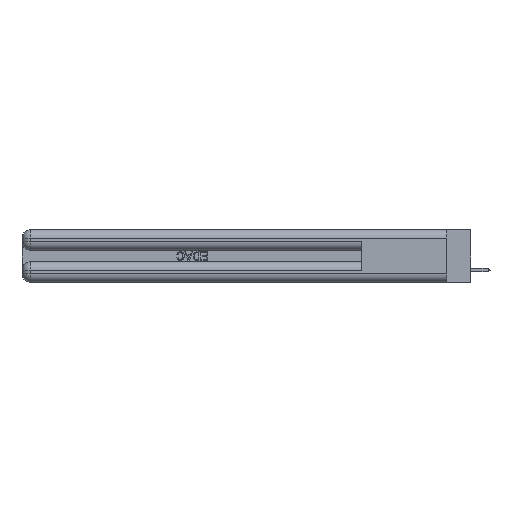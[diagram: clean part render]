
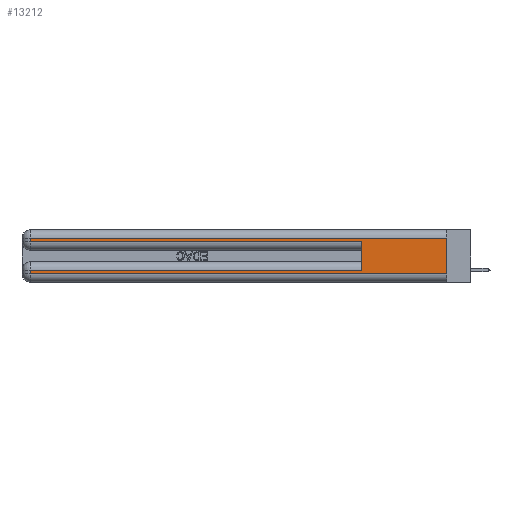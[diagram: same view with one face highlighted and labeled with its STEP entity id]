
A CAD part, left-side view. The second image highlights one B-rep face of the part: STEP entity #13212.
In plain terms, the highlighted planar face has unit normal (-1, 0, 0).
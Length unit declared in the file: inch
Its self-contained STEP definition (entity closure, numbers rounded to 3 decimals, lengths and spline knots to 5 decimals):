
#26 = EDGE_LOOP ( 'NONE', ( #48229, #40978, #5168, #26875, #28088, #43098, #944, #20718 ) ) ;
#944 = ORIENTED_EDGE ( 'NONE', *, *, #6880, .T. ) ;
#1150 = DIRECTION ( 'NONE',  ( 0., 0., -1. ) ) ;
#1987 = VECTOR ( 'NONE', #1150, 39.37008 ) ;
#2063 = EDGE_CURVE ( 'NONE', #20441, #38896, #4569, .T. ) ;
#2819 = EDGE_CURVE ( 'NONE', #20441, #10997, #40983, .T. ) ;
#4569 = LINE ( 'NONE', #18799, #24946 ) ;
#5143 = DIRECTION ( 'NONE',  ( 0., 1., 0. ) ) ;
#5168 = ORIENTED_EDGE ( 'NONE', *, *, #30772, .T. ) ;
#6452 = LINE ( 'NONE', #38888, #9509 ) ;
#6711 = EDGE_CURVE ( 'NONE', #26105, #38896, #39198, .T. ) ;
#6880 = EDGE_CURVE ( 'NONE', #10997, #44248, #21819, .T. ) ;
#7583 = VERTEX_POINT ( 'NONE', #15220 ) ;
#7805 = PLANE ( 'NONE',  #35857 ) ;
#7913 = DIRECTION ( 'NONE',  ( 0., 0., 1. ) ) ;
#7926 = CARTESIAN_POINT ( 'NONE',  ( 0., 2.94, 0.085 ) ) ;
#8089 = DIRECTION ( 'NONE',  ( 0., -1., 0. ) ) ;
#8576 = DIRECTION ( 'NONE',  ( 0., -1., 0. ) ) ;
#9509 = VECTOR ( 'NONE', #20140, 39.37008 ) ;
#10997 = VERTEX_POINT ( 'NONE', #7926 ) ;
#11339 = CARTESIAN_POINT ( 'NONE',  ( 0., 0., 0.31 ) ) ;
#13212 = ADVANCED_FACE ( 'NONE', ( #26856 ), #7805, .F. ) ;
#14032 = CARTESIAN_POINT ( 'NONE',  ( 0., 2.94, 0.285 ) ) ;
#15220 = CARTESIAN_POINT ( 'NONE',  ( 0., 2.94, 0.31 ) ) ;
#18799 = CARTESIAN_POINT ( 'NONE',  ( 0., 0.6, 0.145 ) ) ;
#18947 = VECTOR ( 'NONE', #5143, 39.37008 ) ;
#19953 = LINE ( 'NONE', #28258, #47176 ) ;
#19994 = DIRECTION ( 'NONE',  ( 0., 1., 0. ) ) ;
#20140 = DIRECTION ( 'NONE',  ( 0., 0., -1. ) ) ;
#20441 = VERTEX_POINT ( 'NONE', #39815 ) ;
#20532 = VECTOR ( 'NONE', #19994, 39.37008 ) ;
#20718 = ORIENTED_EDGE ( 'NONE', *, *, #27143, .T. ) ;
#21819 = LINE ( 'NONE', #34352, #29849 ) ;
#22660 = CARTESIAN_POINT ( 'NONE',  ( 0., 2.94, 0.06 ) ) ;
#24946 = VECTOR ( 'NONE', #7913, 39.37008 ) ;
#26105 = VERTEX_POINT ( 'NONE', #14032 ) ;
#26856 = FACE_OUTER_BOUND ( 'NONE', #26, .T. ) ;
#26875 = ORIENTED_EDGE ( 'NONE', *, *, #6711, .T. ) ;
#26922 = EDGE_CURVE ( 'NONE', #35637, #43924, #6452, .T. ) ;
#27143 = EDGE_CURVE ( 'NONE', #44248, #43924, #19953, .T. ) ;
#27499 = DIRECTION ( 'NONE',  ( 0., 0., -1. ) ) ;
#28088 = ORIENTED_EDGE ( 'NONE', *, *, #2063, .F. ) ;
#28258 = CARTESIAN_POINT ( 'NONE',  ( 0., 0., 0.06 ) ) ;
#29849 = VECTOR ( 'NONE', #38376, 39.37008 ) ;
#30772 = EDGE_CURVE ( 'NONE', #7583, #26105, #40287, .T. ) ;
#34352 = CARTESIAN_POINT ( 'NONE',  ( 0., 2.94, 0.37 ) ) ;
#35561 = CARTESIAN_POINT ( 'NONE',  ( 0., 0., 0.285 ) ) ;
#35637 = VERTEX_POINT ( 'NONE', #11339 ) ;
#35857 = AXIS2_PLACEMENT_3D ( 'NONE', #50812, #50976, #27499 ) ;
#37541 = LINE ( 'NONE', #45034, #18947 ) ;
#38376 = DIRECTION ( 'NONE',  ( 0., 0., -1. ) ) ;
#38888 = CARTESIAN_POINT ( 'NONE',  ( 0., 0., 0.37 ) ) ;
#38896 = VERTEX_POINT ( 'NONE', #50313 ) ;
#39198 = LINE ( 'NONE', #35561, #45946 ) ;
#39815 = CARTESIAN_POINT ( 'NONE',  ( 0., 0.6, 0.085 ) ) ;
#40287 = LINE ( 'NONE', #44130, #1987 ) ;
#40659 = CARTESIAN_POINT ( 'NONE',  ( 0., 0., 0.06 ) ) ;
#40978 = ORIENTED_EDGE ( 'NONE', *, *, #41626, .T. ) ;
#40983 = LINE ( 'NONE', #50243, #20532 ) ;
#41626 = EDGE_CURVE ( 'NONE', #35637, #7583, #37541, .T. ) ;
#43098 = ORIENTED_EDGE ( 'NONE', *, *, #2819, .T. ) ;
#43924 = VERTEX_POINT ( 'NONE', #40659 ) ;
#44130 = CARTESIAN_POINT ( 'NONE',  ( 0., 2.94, 0.37 ) ) ;
#44248 = VERTEX_POINT ( 'NONE', #22660 ) ;
#45034 = CARTESIAN_POINT ( 'NONE',  ( 0., 0., 0.31 ) ) ;
#45946 = VECTOR ( 'NONE', #8089, 39.37008 ) ;
#47176 = VECTOR ( 'NONE', #8576, 39.37008 ) ;
#48229 = ORIENTED_EDGE ( 'NONE', *, *, #26922, .F. ) ;
#50243 = CARTESIAN_POINT ( 'NONE',  ( 0., 0., 0.085 ) ) ;
#50313 = CARTESIAN_POINT ( 'NONE',  ( 0., 0.6, 0.285 ) ) ;
#50812 = CARTESIAN_POINT ( 'NONE',  ( 0., 0., 0.37 ) ) ;
#50976 = DIRECTION ( 'NONE',  ( 1., 0., 0. ) ) ;
